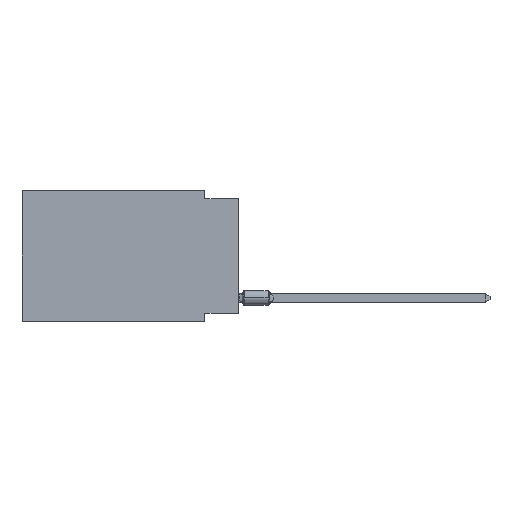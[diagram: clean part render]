
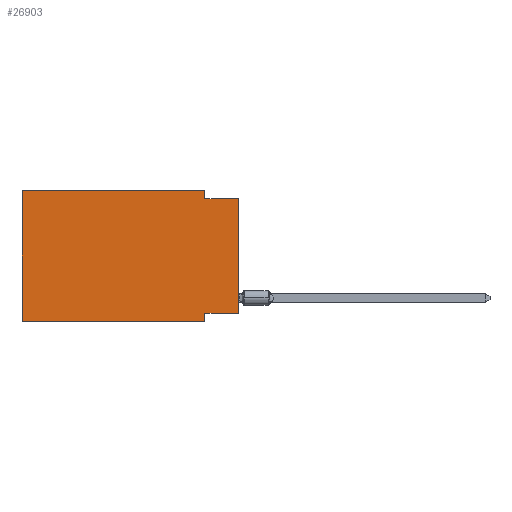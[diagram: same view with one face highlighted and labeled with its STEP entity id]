
A CAD part, left-side view. The second image highlights one B-rep face of the part: STEP entity #26903.
In plain terms, the highlighted planar face has unit normal (-1, 0, 0).
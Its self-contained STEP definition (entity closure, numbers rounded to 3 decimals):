
#568 = EDGE_CURVE ( 'NONE', #10341, #23876, #2651, .T. ) ;
#661 = ORIENTED_EDGE ( 'NONE', *, *, #18958, .F. ) ;
#689 = VERTEX_POINT ( 'NONE', #31804 ) ;
#2224 = EDGE_CURVE ( 'NONE', #15862, #689, #13584, .T. ) ;
#2651 = LINE ( 'NONE', #10770, #17782 ) ;
#2760 = VERTEX_POINT ( 'NONE', #27590 ) ;
#3160 = LINE ( 'NONE', #8739, #8960 ) ;
#3335 = CARTESIAN_POINT ( 'NONE',  ( 0., 16.383, 0. ) ) ;
#3598 = DIRECTION ( 'NONE',  ( 0., -1., 0. ) ) ;
#4628 = VECTOR ( 'NONE', #18805, 1000. ) ;
#6311 = EDGE_CURVE ( 'NONE', #16880, #19415, #19732, .T. ) ;
#6324 = VECTOR ( 'NONE', #31218, 1000. ) ;
#7245 = VECTOR ( 'NONE', #22101, 1000. ) ;
#7306 = DIRECTION ( 'NONE',  ( 0., 0., -1. ) ) ;
#8739 = CARTESIAN_POINT ( 'NONE',  ( 0., 16.383, 0. ) ) ;
#8960 = VECTOR ( 'NONE', #31473, 1000. ) ;
#9197 = DIRECTION ( 'NONE',  ( 0., 1., 0. ) ) ;
#9438 = EDGE_CURVE ( 'NONE', #689, #23876, #10540, .T. ) ;
#9785 = ORIENTED_EDGE ( 'NONE', *, *, #568, .T. ) ;
#9857 = CARTESIAN_POINT ( 'NONE',  ( 0., 16.383, 0. ) ) ;
#10341 = VERTEX_POINT ( 'NONE', #31240 ) ;
#10369 = LINE ( 'NONE', #20304, #19296 ) ;
#10413 = DIRECTION ( 'NONE',  ( 0., 0., 1. ) ) ;
#10540 = LINE ( 'NONE', #26682, #30778 ) ;
#10770 = CARTESIAN_POINT ( 'NONE',  ( 0., 0., 0. ) ) ;
#10952 = ORIENTED_EDGE ( 'NONE', *, *, #20679, .F. ) ;
#12870 = CARTESIAN_POINT ( 'NONE',  ( 0., 2.54, -9.906 ) ) ;
#13147 = CARTESIAN_POINT ( 'NONE',  ( 0., 0., -0.635 ) ) ;
#13341 = AXIS2_PLACEMENT_3D ( 'NONE', #9857, #20121, #7306 ) ;
#13584 = LINE ( 'NONE', #26009, #4628 ) ;
#14169 = EDGE_CURVE ( 'NONE', #10341, #2760, #27525, .T. ) ;
#14191 = CARTESIAN_POINT ( 'NONE',  ( 0., 16.383, -9.906 ) ) ;
#15112 = ORIENTED_EDGE ( 'NONE', *, *, #23454, .F. ) ;
#15862 = VERTEX_POINT ( 'NONE', #22936 ) ;
#16060 = EDGE_LOOP ( 'NONE', ( #9785, #28850, #21535, #15112, #661, #29678, #10952, #27766 ) ) ;
#16534 = CARTESIAN_POINT ( 'NONE',  ( 0., 16.383, -9.906 ) ) ;
#16880 = VERTEX_POINT ( 'NONE', #16534 ) ;
#17782 = VECTOR ( 'NONE', #10413, 1000. ) ;
#17963 = VECTOR ( 'NONE', #9197, 1000. ) ;
#18089 = LINE ( 'NONE', #12870, #6324 ) ;
#18805 = DIRECTION ( 'NONE',  ( 0., 0., -1. ) ) ;
#18958 = EDGE_CURVE ( 'NONE', #16880, #26061, #3160, .T. ) ;
#19296 = VECTOR ( 'NONE', #31078, 1000. ) ;
#19415 = VERTEX_POINT ( 'NONE', #32269 ) ;
#19465 = CARTESIAN_POINT ( 'NONE',  ( 0., 0., -9.271 ) ) ;
#19732 = LINE ( 'NONE', #14191, #7245 ) ;
#20121 = DIRECTION ( 'NONE',  ( 1., 0., 0. ) ) ;
#20304 = CARTESIAN_POINT ( 'NONE',  ( 0., 16.383, 0. ) ) ;
#20679 = EDGE_CURVE ( 'NONE', #2760, #19415, #18089, .T. ) ;
#21535 = ORIENTED_EDGE ( 'NONE', *, *, #2224, .F. ) ;
#22101 = DIRECTION ( 'NONE',  ( 0., -1., 0. ) ) ;
#22653 = FACE_OUTER_BOUND ( 'NONE', #16060, .T. ) ;
#22936 = CARTESIAN_POINT ( 'NONE',  ( 0., 2.54, 0. ) ) ;
#23454 = EDGE_CURVE ( 'NONE', #26061, #15862, #10369, .T. ) ;
#23876 = VERTEX_POINT ( 'NONE', #13147 ) ;
#26009 = CARTESIAN_POINT ( 'NONE',  ( 0., 2.54, 0. ) ) ;
#26061 = VERTEX_POINT ( 'NONE', #3335 ) ;
#26682 = CARTESIAN_POINT ( 'NONE',  ( 0., 0., -0.635 ) ) ;
#26903 = ADVANCED_FACE ( 'NONE', ( #22653 ), #32937, .F. ) ;
#27525 = LINE ( 'NONE', #19465, #17963 ) ;
#27590 = CARTESIAN_POINT ( 'NONE',  ( 0., 2.54, -9.271 ) ) ;
#27766 = ORIENTED_EDGE ( 'NONE', *, *, #14169, .F. ) ;
#28850 = ORIENTED_EDGE ( 'NONE', *, *, #9438, .F. ) ;
#29678 = ORIENTED_EDGE ( 'NONE', *, *, #6311, .T. ) ;
#30778 = VECTOR ( 'NONE', #3598, 1000. ) ;
#31078 = DIRECTION ( 'NONE',  ( 0., -1., 0. ) ) ;
#31218 = DIRECTION ( 'NONE',  ( 0., 0., -1. ) ) ;
#31240 = CARTESIAN_POINT ( 'NONE',  ( 0., 0., -9.271 ) ) ;
#31473 = DIRECTION ( 'NONE',  ( 0., 0., 1. ) ) ;
#31804 = CARTESIAN_POINT ( 'NONE',  ( 0., 2.54, -0.635 ) ) ;
#32269 = CARTESIAN_POINT ( 'NONE',  ( 0., 2.54, -9.906 ) ) ;
#32937 = PLANE ( 'NONE',  #13341 ) ;
